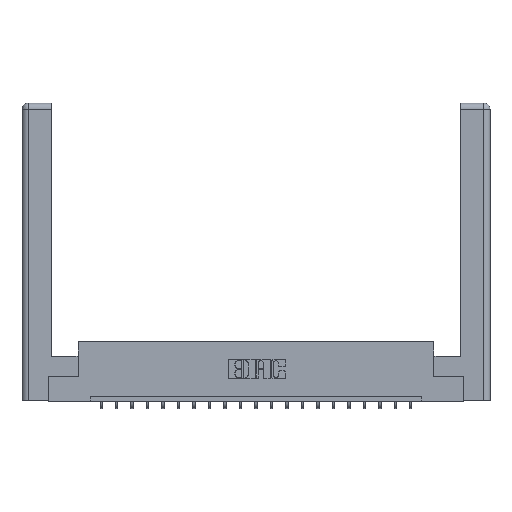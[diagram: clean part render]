
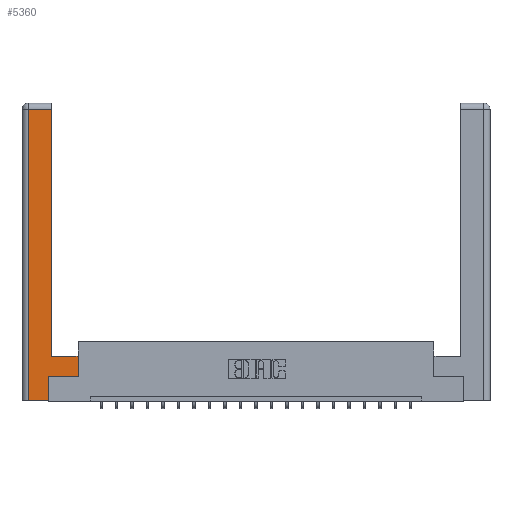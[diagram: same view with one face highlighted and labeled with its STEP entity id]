
A CAD part, top view. The second image highlights one B-rep face of the part: STEP entity #5360.
In plain terms, the highlighted planar face has unit normal (0, 0, 1).
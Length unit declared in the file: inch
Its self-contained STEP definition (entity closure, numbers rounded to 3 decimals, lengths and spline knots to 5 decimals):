
#129 = LINE ( 'NONE', #14616, #11827 ) ;
#254 = CARTESIAN_POINT ( 'NONE',  ( 0.265, 0.245, 0. ) ) ;
#725 = EDGE_CURVE ( 'NONE', #2291, #13313, #6323, .T. ) ;
#997 = VECTOR ( 'NONE', #11167, 39.37008 ) ;
#1301 = VECTOR ( 'NONE', #8776, 39.37008 ) ;
#1791 = LINE ( 'NONE', #15831, #4348 ) ;
#2291 = VERTEX_POINT ( 'NONE', #6597 ) ;
#3062 = CARTESIAN_POINT ( 'NONE',  ( 0.0615, 2.94, 0. ) ) ;
#3554 = LINE ( 'NONE', #7908, #997 ) ;
#3680 = VECTOR ( 'NONE', #6354, 39.37008 ) ;
#3890 = CARTESIAN_POINT ( 'NONE',  ( 0., 0., 0. ) ) ;
#3898 = EDGE_CURVE ( 'NONE', #20744, #20053, #1791, .T. ) ;
#3949 = ORIENTED_EDGE ( 'NONE', *, *, #13767, .T. ) ;
#4254 = CARTESIAN_POINT ( 'NONE',  ( 0.295, 3., 0. ) ) ;
#4348 = VECTOR ( 'NONE', #17520, 39.37008 ) ;
#4624 = DIRECTION ( 'NONE',  ( -1., 0., 0. ) ) ;
#4664 = ORIENTED_EDGE ( 'NONE', *, *, #11983, .T. ) ;
#4725 = CARTESIAN_POINT ( 'NONE',  ( 0.295, 0.45, 0. ) ) ;
#5055 = DIRECTION ( 'NONE',  ( 1., 0., 0. ) ) ;
#5276 = CARTESIAN_POINT ( 'NONE',  ( 0.295, 0.45, 0. ) ) ;
#5360 = ADVANCED_FACE ( 'NONE', ( #17237 ), #17021, .F. ) ;
#5572 = VECTOR ( 'NONE', #4624, 39.37008 ) ;
#5640 = LINE ( 'NONE', #4254, #1301 ) ;
#5923 = ORIENTED_EDGE ( 'NONE', *, *, #8415, .T. ) ;
#5981 = CARTESIAN_POINT ( 'NONE',  ( 0.0615, 0., 0. ) ) ;
#6065 = CARTESIAN_POINT ( 'NONE',  ( 0.565, 0.45, 0. ) ) ;
#6142 = ORIENTED_EDGE ( 'NONE', *, *, #11663, .T. ) ;
#6323 = LINE ( 'NONE', #3062, #5572 ) ;
#6354 = DIRECTION ( 'NONE',  ( -1., 0., 0. ) ) ;
#6597 = CARTESIAN_POINT ( 'NONE',  ( 0.295, 2.94, 0. ) ) ;
#7051 = CARTESIAN_POINT ( 'NONE',  ( 0.565, 0.245, 0. ) ) ;
#7908 = CARTESIAN_POINT ( 'NONE',  ( 0.0615, 0., 0. ) ) ;
#8172 = VERTEX_POINT ( 'NONE', #5276 ) ;
#8415 = EDGE_CURVE ( 'NONE', #8172, #2291, #5640, .T. ) ;
#8776 = DIRECTION ( 'NONE',  ( 0., 1., 0. ) ) ;
#8855 = DIRECTION ( 'NONE',  ( -1., 0., 0. ) ) ;
#9064 = CARTESIAN_POINT ( 'NONE',  ( 0.565, 0.45, 0. ) ) ;
#10433 = DIRECTION ( 'NONE',  ( 0., 0., -1. ) ) ;
#10529 = LINE ( 'NONE', #254, #11282 ) ;
#10955 = VERTEX_POINT ( 'NONE', #6065 ) ;
#11167 = DIRECTION ( 'NONE',  ( 0., -1., 0. ) ) ;
#11282 = VECTOR ( 'NONE', #11627, 39.37008 ) ;
#11627 = DIRECTION ( 'NONE',  ( 0., 1., 0. ) ) ;
#11663 = EDGE_CURVE ( 'NONE', #17081, #16391, #129, .T. ) ;
#11827 = VECTOR ( 'NONE', #5055, 39.37008 ) ;
#11983 = EDGE_CURVE ( 'NONE', #10955, #8172, #20200, .T. ) ;
#12947 = VECTOR ( 'NONE', #20501, 39.37008 ) ;
#13313 = VERTEX_POINT ( 'NONE', #14739 ) ;
#13767 = EDGE_CURVE ( 'NONE', #16391, #20744, #10529, .T. ) ;
#14616 = CARTESIAN_POINT ( 'NONE',  ( 0.265, 0., 0. ) ) ;
#14739 = CARTESIAN_POINT ( 'NONE',  ( 0.0615, 2.94, 0. ) ) ;
#15714 = LINE ( 'NONE', #9064, #12947 ) ;
#15796 = ORIENTED_EDGE ( 'NONE', *, *, #16375, .T. ) ;
#15831 = CARTESIAN_POINT ( 'NONE',  ( 0.565, 0.245, 0. ) ) ;
#15936 = CARTESIAN_POINT ( 'NONE',  ( 0.265, 0.245, 0. ) ) ;
#16294 = ORIENTED_EDGE ( 'NONE', *, *, #16985, .T. ) ;
#16375 = EDGE_CURVE ( 'NONE', #20053, #10955, #15714, .T. ) ;
#16391 = VERTEX_POINT ( 'NONE', #20437 ) ;
#16985 = EDGE_CURVE ( 'NONE', #13313, #17081, #3554, .T. ) ;
#17021 = PLANE ( 'NONE',  #17399 ) ;
#17081 = VERTEX_POINT ( 'NONE', #5981 ) ;
#17237 = FACE_OUTER_BOUND ( 'NONE', #21030, .T. ) ;
#17399 = AXIS2_PLACEMENT_3D ( 'NONE', #3890, #10433, #8855 ) ;
#17406 = ORIENTED_EDGE ( 'NONE', *, *, #725, .T. ) ;
#17520 = DIRECTION ( 'NONE',  ( 1., 0., 0. ) ) ;
#20053 = VERTEX_POINT ( 'NONE', #7051 ) ;
#20105 = ORIENTED_EDGE ( 'NONE', *, *, #3898, .T. ) ;
#20200 = LINE ( 'NONE', #4725, #3680 ) ;
#20437 = CARTESIAN_POINT ( 'NONE',  ( 0.265, 0., 0. ) ) ;
#20501 = DIRECTION ( 'NONE',  ( 0., 1., 0. ) ) ;
#20744 = VERTEX_POINT ( 'NONE', #15936 ) ;
#21030 = EDGE_LOOP ( 'NONE', ( #5923, #17406, #16294, #6142, #3949, #20105, #15796, #4664 ) ) ;
